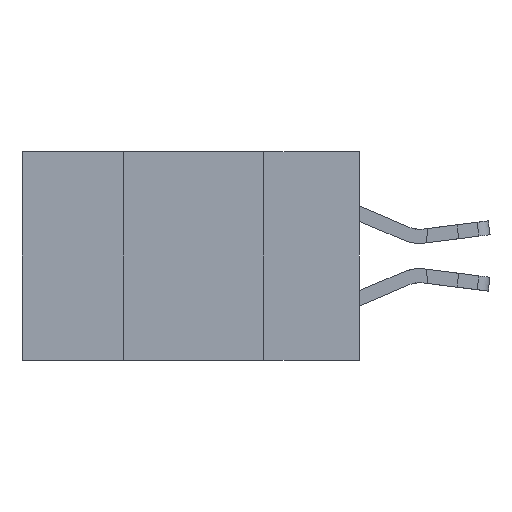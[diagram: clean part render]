
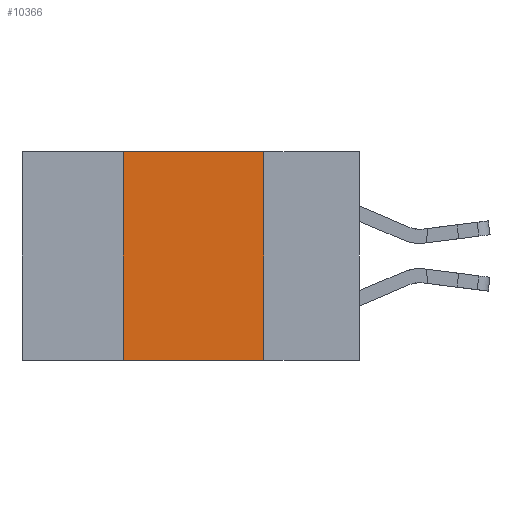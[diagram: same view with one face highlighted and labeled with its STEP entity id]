
A CAD part, left-side view. The second image highlights one B-rep face of the part: STEP entity #10366.
In plain terms, the highlighted planar face has unit normal (-1, 0, 0).
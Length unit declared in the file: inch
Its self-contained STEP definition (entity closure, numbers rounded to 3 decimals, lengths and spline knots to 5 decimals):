
#677 = PLANE ( 'NONE',  #9219 ) ;
#1146 = ORIENTED_EDGE ( 'NONE', *, *, #12462, .T. ) ;
#1621 = DIRECTION ( 'NONE',  ( 0., 0., 1. ) ) ;
#1902 = VERTEX_POINT ( 'NONE', #6156 ) ;
#2090 = CARTESIAN_POINT ( 'NONE',  ( 0., 0.17, 0. ) ) ;
#2109 = DIRECTION ( 'NONE',  ( 0., 0., -1. ) ) ;
#2475 = LINE ( 'NONE', #11063, #16847 ) ;
#2840 = CARTESIAN_POINT ( 'NONE',  ( 0., 0.6, 0. ) ) ;
#3215 = FACE_OUTER_BOUND ( 'NONE', #12517, .T. ) ;
#6156 = CARTESIAN_POINT ( 'NONE',  ( 0., 0.42, 0. ) ) ;
#6236 = CARTESIAN_POINT ( 'NONE',  ( 0., 0.6, 0. ) ) ;
#6884 = VERTEX_POINT ( 'NONE', #13345 ) ;
#7652 = VECTOR ( 'NONE', #13211, 39.37008 ) ;
#9219 = AXIS2_PLACEMENT_3D ( 'NONE', #6236, #10184, #2109 ) ;
#10184 = DIRECTION ( 'NONE',  ( 1., 0., 0. ) ) ;
#10366 = ADVANCED_FACE ( 'NONE', ( #3215 ), #677, .F. ) ;
#10501 = CARTESIAN_POINT ( 'NONE',  ( 0., 0.42, -0.37 ) ) ;
#10617 = VERTEX_POINT ( 'NONE', #14459 ) ;
#10669 = ORIENTED_EDGE ( 'NONE', *, *, #15083, .F. ) ;
#10835 = DIRECTION ( 'NONE',  ( 0., -1., 0. ) ) ;
#11063 = CARTESIAN_POINT ( 'NONE',  ( 0., 0.42, 0. ) ) ;
#11112 = LINE ( 'NONE', #16990, #7652 ) ;
#11638 = LINE ( 'NONE', #2840, #14232 ) ;
#12150 = ORIENTED_EDGE ( 'NONE', *, *, #14196, .F. ) ;
#12360 = VERTEX_POINT ( 'NONE', #10501 ) ;
#12462 = EDGE_CURVE ( 'NONE', #12360, #6884, #11112, .T. ) ;
#12517 = EDGE_LOOP ( 'NONE', ( #10669, #16922, #12150, #1146 ) ) ;
#12723 = DIRECTION ( 'NONE',  ( 0., 0., -1. ) ) ;
#12982 = LINE ( 'NONE', #2090, #13384 ) ;
#13211 = DIRECTION ( 'NONE',  ( 0., -1., 0. ) ) ;
#13345 = CARTESIAN_POINT ( 'NONE',  ( 0., 0.17, -0.37 ) ) ;
#13384 = VECTOR ( 'NONE', #12723, 39.37008 ) ;
#14091 = EDGE_CURVE ( 'NONE', #1902, #10617, #11638, .T. ) ;
#14196 = EDGE_CURVE ( 'NONE', #12360, #1902, #2475, .T. ) ;
#14232 = VECTOR ( 'NONE', #10835, 39.37008 ) ;
#14459 = CARTESIAN_POINT ( 'NONE',  ( 0., 0.17, 0. ) ) ;
#15083 = EDGE_CURVE ( 'NONE', #10617, #6884, #12982, .T. ) ;
#16847 = VECTOR ( 'NONE', #1621, 39.37008 ) ;
#16922 = ORIENTED_EDGE ( 'NONE', *, *, #14091, .F. ) ;
#16990 = CARTESIAN_POINT ( 'NONE',  ( 0., 0.6, -0.37 ) ) ;
